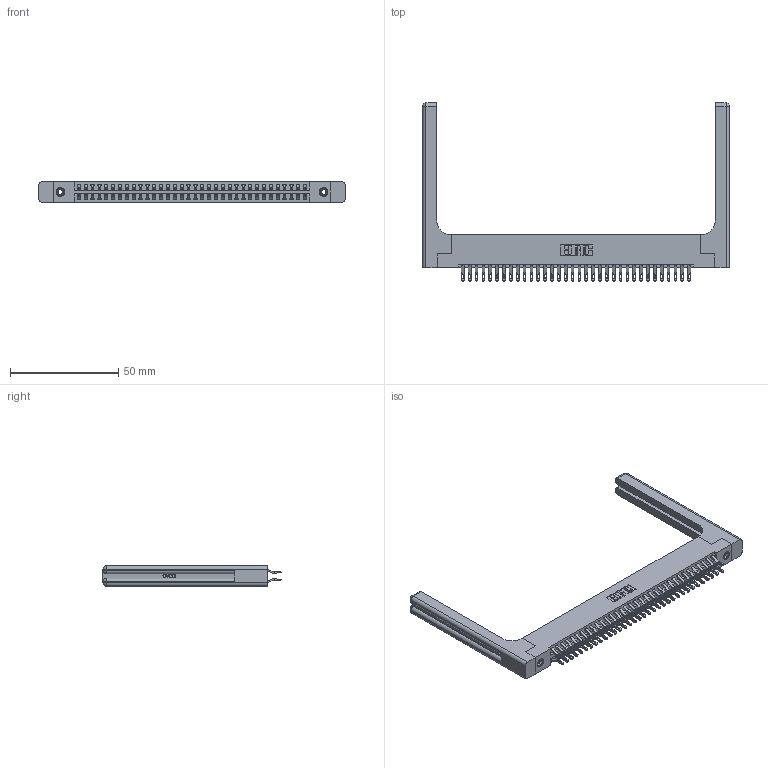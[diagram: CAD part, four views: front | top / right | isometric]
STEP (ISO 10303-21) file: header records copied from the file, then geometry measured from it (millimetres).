
FILE_DESCRIPTION (( 'STEP AP203' ), '1' );
FILE_NAME ('396-068-555-258.STEP', '2019-10-30T19:02:02', ( '' ), ( '' ), 'SwSTEP 2.0', 'SolidWorks 2016', '' );
FILE_SCHEMA (( 'CONFIG_CONTROL_DESIGN' ));
Length unit declared in the file: inch
Products named in the file (5): 345-250-001_345-250-001-102; 346 Part_Flush Mounting Lugs - 0.156 Dia-TH; 345-292-001_555 Tail; 396-068-555-258; 346-220-058_345-220-058
Assembly tree (73 placements, depth 2):
  396-068-555-258
    346 Part_Flush Mounting Lugs - 0.156 Dia-TH
    345-292-001_555 Tail  x68
    345-250-001_345-250-001-102  x2
    346-220-058_345-220-058  x2
Bounding box: 142.01 x 82.42 x 9.4 mm (x, y, z)
Volume: 21477.2 mm3; surface area: 24770.7 mm2
Topology: 73 solids, 73 shells, 4322 faces, 13439 edges, 8938 vertices
Faces by surface type: plane 2468, cylinder 1794, bspline 36, cone 12, sphere 8, torus 4
Entity records: 28774 total; most frequent: CARTESIAN_POINT 5795, ORIENTED_EDGE 4496, DIRECTION 4060, EDGE_CURVE 2248, VECTOR 1868, LINE 1868, VERTEX_POINT 1490, AXIS2_PLACEMENT_3D 1096
